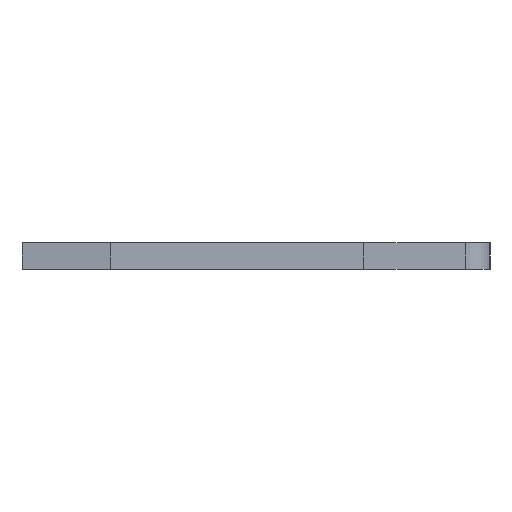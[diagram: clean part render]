
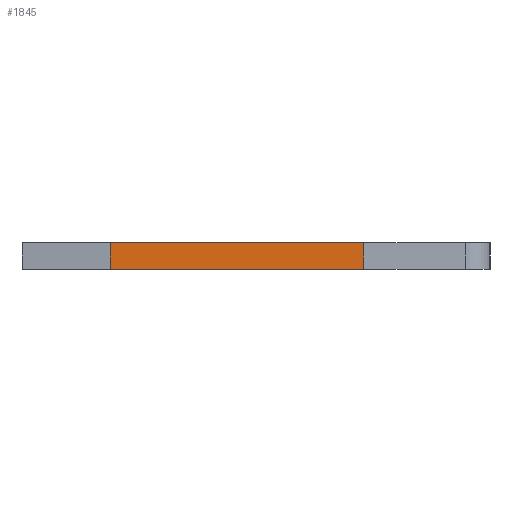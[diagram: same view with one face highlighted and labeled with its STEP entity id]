
A CAD part, left-side view. The second image highlights one B-rep face of the part: STEP entity #1845.
In plain terms, the highlighted face is planar.
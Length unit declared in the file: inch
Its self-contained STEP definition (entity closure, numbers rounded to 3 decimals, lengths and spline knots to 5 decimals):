
#93 = ORIENTED_EDGE ( 'NONE', *, *, #151, .F. ) ;
#132 = ORIENTED_EDGE ( 'NONE', *, *, #754, .T. ) ;
#137 = VERTEX_POINT ( 'NONE', #1147 ) ;
#151 = EDGE_CURVE ( 'NONE', #907, #1499, #1419, .T. ) ;
#160 = EDGE_CURVE ( 'NONE', #137, #619, #1259, .T. ) ;
#293 = EDGE_CURVE ( 'NONE', #1499, #619, #883, .T. ) ;
#336 = DIRECTION ( 'NONE',  ( 0., 0., 1. ) ) ;
#354 = DIRECTION ( 'NONE',  ( -1., 0., 0. ) ) ;
#358 = DIRECTION ( 'NONE',  ( 1., 0., 0. ) ) ;
#471 = CARTESIAN_POINT ( 'NONE',  ( 0.013, 0.146, -0.0575 ) ) ;
#488 = EDGE_LOOP ( 'NONE', ( #946, #1555, #93, #132 ) ) ;
#564 = CARTESIAN_POINT ( 'NONE',  ( 0.013, 0.146, -0.0575 ) ) ;
#611 = PLANE ( 'NONE',  #1016 ) ;
#613 = DIRECTION ( 'NONE',  ( -1., 0., 0. ) ) ;
#619 = VERTEX_POINT ( 'NONE', #620 ) ;
#620 = CARTESIAN_POINT ( 'NONE',  ( -0.013, 0.146, -0.0575 ) ) ;
#639 = CARTESIAN_POINT ( 'NONE',  ( 0.013, -0.099, -0.0575 ) ) ;
#707 = DIRECTION ( 'NONE',  ( 0., 1., 0. ) ) ;
#754 = EDGE_CURVE ( 'NONE', #907, #137, #856, .T. ) ;
#759 = VECTOR ( 'NONE', #707, 39.37008 ) ;
#801 = CARTESIAN_POINT ( 'NONE',  ( 0.013, 0.146, -0.0575 ) ) ;
#856 = LINE ( 'NONE', #639, #1737 ) ;
#869 = CARTESIAN_POINT ( 'NONE',  ( -0.013, 0.146, -0.0575 ) ) ;
#883 = LINE ( 'NONE', #471, #1190 ) ;
#907 = VERTEX_POINT ( 'NONE', #1398 ) ;
#917 = CARTESIAN_POINT ( 'NONE',  ( 0.013, 0.146, -0.0575 ) ) ;
#946 = ORIENTED_EDGE ( 'NONE', *, *, #160, .T. ) ;
#1016 = AXIS2_PLACEMENT_3D ( 'NONE', #917, #336, #358 ) ;
#1147 = CARTESIAN_POINT ( 'NONE',  ( -0.013, -0.099, -0.0575 ) ) ;
#1185 = VECTOR ( 'NONE', #1209, 39.37008 ) ;
#1190 = VECTOR ( 'NONE', #613, 39.37008 ) ;
#1209 = DIRECTION ( 'NONE',  ( 0., 1., 0. ) ) ;
#1259 = LINE ( 'NONE', #869, #759 ) ;
#1398 = CARTESIAN_POINT ( 'NONE',  ( 0.013, -0.099, -0.0575 ) ) ;
#1419 = LINE ( 'NONE', #801, #1185 ) ;
#1499 = VERTEX_POINT ( 'NONE', #564 ) ;
#1555 = ORIENTED_EDGE ( 'NONE', *, *, #293, .F. ) ;
#1615 = FACE_OUTER_BOUND ( 'NONE', #488, .T. ) ;
#1737 = VECTOR ( 'NONE', #354, 39.37008 ) ;
#1845 = ADVANCED_FACE ( 'NONE', ( #1615 ), #611, .F. ) ;
